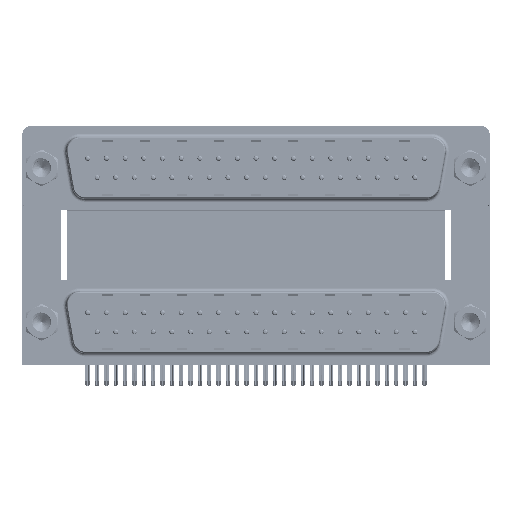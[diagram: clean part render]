
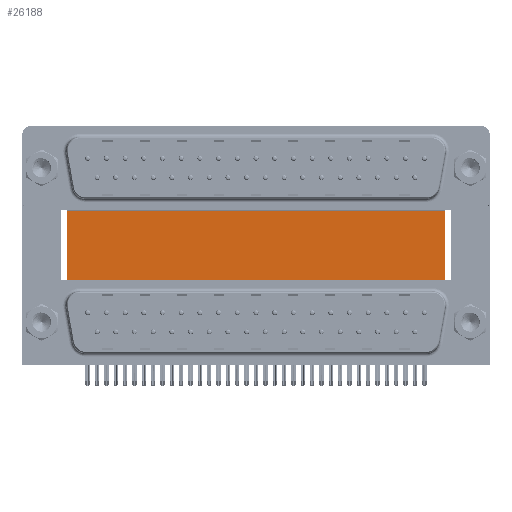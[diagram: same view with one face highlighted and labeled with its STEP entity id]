
A CAD part, top view. The second image highlights one B-rep face of the part: STEP entity #26188.
In plain terms, the highlighted planar face has unit normal (0, 0, 1).
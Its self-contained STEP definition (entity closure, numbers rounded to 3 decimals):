
#1477 = CARTESIAN_POINT ( 'NONE',  ( 59.71, -3.735, -12. ) ) ;
#3260 = CARTESIAN_POINT ( 'NONE',  ( 3.79, 16.585, -12. ) ) ;
#3535 = LINE ( 'NONE', #16789, #37130 ) ;
#5874 = CARTESIAN_POINT ( 'NONE',  ( 3.79, 16.585, -12. ) ) ;
#7384 = FACE_OUTER_BOUND ( 'NONE', #49979, .T. ) ;
#8248 = ORIENTED_EDGE ( 'NONE', *, *, #15836, .T. ) ;
#11512 = VECTOR ( 'NONE', #27053, 1000. ) ;
#11960 = EDGE_CURVE ( 'NONE', #32772, #49444, #18249, .T. ) ;
#14392 = DIRECTION ( 'NONE',  ( 0., -1., 0. ) ) ;
#15836 = EDGE_CURVE ( 'NONE', #41321, #24665, #54636, .T. ) ;
#16499 = DIRECTION ( 'NONE',  ( 1., 0., 0. ) ) ;
#16789 = CARTESIAN_POINT ( 'NONE',  ( 3.79, 16.585, -12. ) ) ;
#18249 = LINE ( 'NONE', #57917, #11512 ) ;
#19817 = VECTOR ( 'NONE', #14392, 1000. ) ;
#20127 = EDGE_CURVE ( 'NONE', #24665, #49444, #26601, .T. ) ;
#21434 = ORIENTED_EDGE ( 'NONE', *, *, #39721, .F. ) ;
#23500 = CARTESIAN_POINT ( 'NONE',  ( 3.79, -3.735, -12. ) ) ;
#24665 = VERTEX_POINT ( 'NONE', #23500 ) ;
#26187 = DIRECTION ( 'NONE',  ( 0., 0., -1. ) ) ;
#26188 = ADVANCED_FACE ( 'NONE', ( #7384 ), #30583, .F. ) ;
#26601 = LINE ( 'NONE', #35978, #48318 ) ;
#27053 = DIRECTION ( 'NONE',  ( 0., -1., 0. ) ) ;
#30583 = PLANE ( 'NONE',  #53342 ) ;
#32772 = VERTEX_POINT ( 'NONE', #43307 ) ;
#35978 = CARTESIAN_POINT ( 'NONE',  ( 3.79, -3.735, -12. ) ) ;
#37130 = VECTOR ( 'NONE', #16499, 1000. ) ;
#39721 = EDGE_CURVE ( 'NONE', #41321, #32772, #3535, .T. ) ;
#41321 = VERTEX_POINT ( 'NONE', #5874 ) ;
#43307 = CARTESIAN_POINT ( 'NONE',  ( 59.71, 16.585, -12. ) ) ;
#46107 = CARTESIAN_POINT ( 'NONE',  ( 3.79, 16.585, -12. ) ) ;
#48318 = VECTOR ( 'NONE', #53326, 1000. ) ;
#48812 = ORIENTED_EDGE ( 'NONE', *, *, #11960, .F. ) ;
#49444 = VERTEX_POINT ( 'NONE', #1477 ) ;
#49979 = EDGE_LOOP ( 'NONE', ( #54837, #48812, #21434, #8248 ) ) ;
#52915 = DIRECTION ( 'NONE',  ( -1., 0., 0. ) ) ;
#53326 = DIRECTION ( 'NONE',  ( 1., 0., 0. ) ) ;
#53342 = AXIS2_PLACEMENT_3D ( 'NONE', #3260, #26187, #52915 ) ;
#54636 = LINE ( 'NONE', #46107, #19817 ) ;
#54837 = ORIENTED_EDGE ( 'NONE', *, *, #20127, .T. ) ;
#57917 = CARTESIAN_POINT ( 'NONE',  ( 59.71, 16.585, -12. ) ) ;
